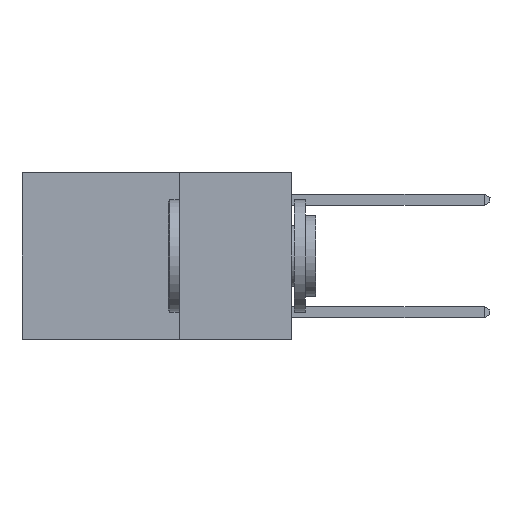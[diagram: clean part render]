
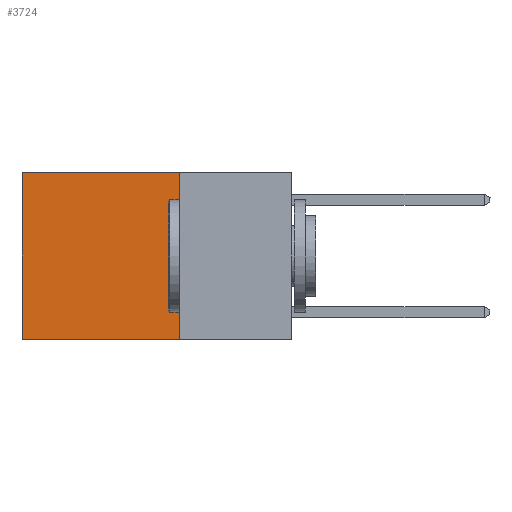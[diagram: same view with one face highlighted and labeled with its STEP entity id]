
A CAD part, left-side view. The second image highlights one B-rep face of the part: STEP entity #3724.
In plain terms, the highlighted planar face has unit normal (-1, 0, 0).
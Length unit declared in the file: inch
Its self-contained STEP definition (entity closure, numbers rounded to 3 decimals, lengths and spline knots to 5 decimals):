
#905 = EDGE_CURVE ( 'NONE', #13335, #4915, #14781, .T. ) ;
#1498 = PLANE ( 'NONE',  #6909 ) ;
#2013 = DIRECTION ( 'NONE',  ( 0., 0., -1. ) ) ;
#3720 = ORIENTED_EDGE ( 'NONE', *, *, #905, .T. ) ;
#3724 = ADVANCED_FACE ( 'NONE', ( #13565 ), #1498, .F. ) ;
#3989 = ORIENTED_EDGE ( 'NONE', *, *, #8908, .F. ) ;
#4327 = ORIENTED_EDGE ( 'NONE', *, *, #12849, .T. ) ;
#4576 = DIRECTION ( 'NONE',  ( 0., 1., 0. ) ) ;
#4756 = CARTESIAN_POINT ( 'NONE',  ( 0.2625, 0.25, -0.37 ) ) ;
#4915 = VERTEX_POINT ( 'NONE', #14083 ) ;
#5735 = VERTEX_POINT ( 'NONE', #19212 ) ;
#6322 = CARTESIAN_POINT ( 'NONE',  ( 0.2625, 0.25, -0.37 ) ) ;
#6909 = AXIS2_PLACEMENT_3D ( 'NONE', #8674, #8450, #8330 ) ;
#7887 = EDGE_LOOP ( 'NONE', ( #3720, #3989, #22081, #4327 ) ) ;
#8214 = VECTOR ( 'NONE', #2013, 39.37008 ) ;
#8330 = DIRECTION ( 'NONE',  ( 0., 0., -1. ) ) ;
#8450 = DIRECTION ( 'NONE',  ( 1., 0., 0. ) ) ;
#8636 = LINE ( 'NONE', #15874, #13291 ) ;
#8674 = CARTESIAN_POINT ( 'NONE',  ( 0.2625, 0.25, 0. ) ) ;
#8908 = EDGE_CURVE ( 'NONE', #11094, #4915, #15913, .T. ) ;
#11094 = VERTEX_POINT ( 'NONE', #4756 ) ;
#12849 = EDGE_CURVE ( 'NONE', #5735, #13335, #20390, .T. ) ;
#13291 = VECTOR ( 'NONE', #23082, 39.37008 ) ;
#13335 = VERTEX_POINT ( 'NONE', #15608 ) ;
#13565 = FACE_OUTER_BOUND ( 'NONE', #7887, .T. ) ;
#14083 = CARTESIAN_POINT ( 'NONE',  ( 0.2625, 0.6, -0.37 ) ) ;
#14427 = EDGE_CURVE ( 'NONE', #5735, #11094, #8636, .T. ) ;
#14781 = LINE ( 'NONE', #16685, #8214 ) ;
#15608 = CARTESIAN_POINT ( 'NONE',  ( 0.2625, 0.6, 0. ) ) ;
#15874 = CARTESIAN_POINT ( 'NONE',  ( 0.2625, 0.25, 0. ) ) ;
#15913 = LINE ( 'NONE', #6322, #16185 ) ;
#16185 = VECTOR ( 'NONE', #4576, 39.37008 ) ;
#16685 = CARTESIAN_POINT ( 'NONE',  ( 0.2625, 0.6, 0. ) ) ;
#17420 = CARTESIAN_POINT ( 'NONE',  ( 0.2625, 0.25, 0. ) ) ;
#18843 = DIRECTION ( 'NONE',  ( 0., 1., 0. ) ) ;
#19212 = CARTESIAN_POINT ( 'NONE',  ( 0.2625, 0.25, 0. ) ) ;
#20390 = LINE ( 'NONE', #17420, #21544 ) ;
#21544 = VECTOR ( 'NONE', #18843, 39.37008 ) ;
#22081 = ORIENTED_EDGE ( 'NONE', *, *, #14427, .F. ) ;
#23082 = DIRECTION ( 'NONE',  ( 0., 0., -1. ) ) ;
